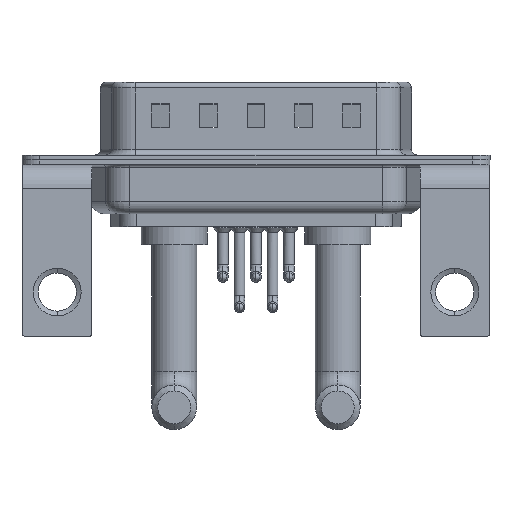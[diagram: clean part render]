
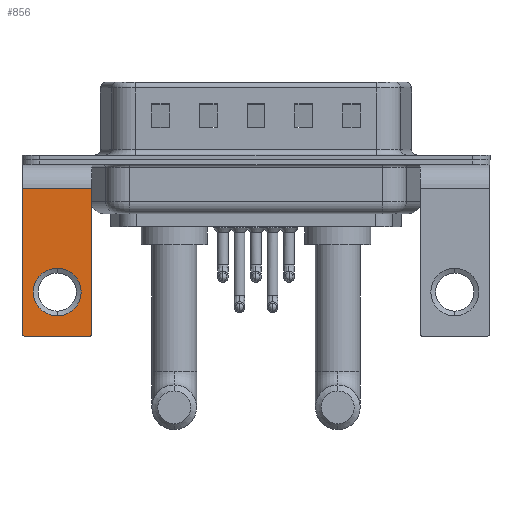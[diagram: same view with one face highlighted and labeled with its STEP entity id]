
A CAD part, front view. The second image highlights one B-rep face of the part: STEP entity #856.
In plain terms, the highlighted planar face has unit normal (0, -1, 0).
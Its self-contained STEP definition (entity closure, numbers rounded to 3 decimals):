
#97 = CARTESIAN_POINT ( 'NONE',  ( -2.65, -6.25, -14.55 ) ) ;
#414 = AXIS2_PLACEMENT_3D ( 'NONE', #17621, #9198, #20740 ) ;
#856 = ADVANCED_FACE ( 'NONE', ( #18692, #6859 ), #3530, .F. ) ;
#1128 = LINE ( 'NONE', #6307, #4351 ) ;
#1333 = EDGE_CURVE ( 'NONE', #2789, #5580, #4740, .T. ) ;
#2203 = DIRECTION ( 'NONE',  ( 0., 0., -1. ) ) ;
#2789 = VERTEX_POINT ( 'NONE', #12906 ) ;
#2883 = CARTESIAN_POINT ( 'NONE',  ( 2.65, -6.25, -14.55 ) ) ;
#3530 = PLANE ( 'NONE',  #4388 ) ;
#3622 = DIRECTION ( 'NONE',  ( 0., -1., 0. ) ) ;
#3652 = DIRECTION ( 'NONE',  ( 0., 0., 1. ) ) ;
#4194 = CARTESIAN_POINT ( 'NONE',  ( 0., -6.25, -11.07 ) ) ;
#4195 = CARTESIAN_POINT ( 'NONE',  ( 2.65, -6.25, -14.8 ) ) ;
#4351 = VECTOR ( 'NONE', #12850, 1000. ) ;
#4388 = AXIS2_PLACEMENT_3D ( 'NONE', #10601, #6972, #3652 ) ;
#4590 = CARTESIAN_POINT ( 'NONE',  ( 0., -6.25, -13.07 ) ) ;
#4740 = CIRCLE ( 'NONE', #16411, 0.25 ) ;
#4962 = EDGE_CURVE ( 'NONE', #6471, #11011, #20034, .T. ) ;
#5580 = VERTEX_POINT ( 'NONE', #7177 ) ;
#5656 = VECTOR ( 'NONE', #13497, 1000. ) ;
#5809 = VERTEX_POINT ( 'NONE', #4590 ) ;
#5896 = ORIENTED_EDGE ( 'NONE', *, *, #1333, .T. ) ;
#6063 = DIRECTION ( 'NONE',  ( 0., 1., 0. ) ) ;
#6274 = ORIENTED_EDGE ( 'NONE', *, *, #7810, .T. ) ;
#6307 = CARTESIAN_POINT ( 'NONE',  ( 2.9, -6.25, -14.8 ) ) ;
#6374 = CIRCLE ( 'NONE', #11019, 0.25 ) ;
#6471 = VERTEX_POINT ( 'NONE', #13721 ) ;
#6859 = FACE_OUTER_BOUND ( 'NONE', #13781, .T. ) ;
#6972 = DIRECTION ( 'NONE',  ( 0., 1., 0. ) ) ;
#7177 = CARTESIAN_POINT ( 'NONE',  ( -2.65, -6.25, -14.8 ) ) ;
#7543 = DIRECTION ( 'NONE',  ( 0., 0., 1. ) ) ;
#7599 = ORIENTED_EDGE ( 'NONE', *, *, #4962, .T. ) ;
#7730 = CARTESIAN_POINT ( 'NONE',  ( 2.9, -6.25, -14.55 ) ) ;
#7810 = EDGE_CURVE ( 'NONE', #20673, #5809, #17030, .T. ) ;
#8917 = DIRECTION ( 'NONE',  ( 0., 0., 1. ) ) ;
#9020 = EDGE_LOOP ( 'NONE', ( #14146, #6274 ) ) ;
#9198 = DIRECTION ( 'NONE',  ( 0., 1., 0. ) ) ;
#9271 = LINE ( 'NONE', #20586, #17512 ) ;
#9598 = DIRECTION ( 'NONE',  ( 0., 0., 1. ) ) ;
#10452 = AXIS2_PLACEMENT_3D ( 'NONE', #4194, #6063, #9598 ) ;
#10601 = CARTESIAN_POINT ( 'NONE',  ( 2.9, -6.25, -2.4 ) ) ;
#11011 = VERTEX_POINT ( 'NONE', #17751 ) ;
#11019 = AXIS2_PLACEMENT_3D ( 'NONE', #2883, #21381, #7543 ) ;
#11727 = CARTESIAN_POINT ( 'NONE',  ( 2.9, -6.25, -2.4 ) ) ;
#11760 = EDGE_CURVE ( 'NONE', #17559, #5580, #1128, .T. ) ;
#11994 = DIRECTION ( 'NONE',  ( 0., 0., -1. ) ) ;
#12850 = DIRECTION ( 'NONE',  ( -1., 0., 0. ) ) ;
#12906 = CARTESIAN_POINT ( 'NONE',  ( -2.9, -6.25, -14.55 ) ) ;
#13293 = EDGE_CURVE ( 'NONE', #11011, #2789, #13332, .T. ) ;
#13332 = LINE ( 'NONE', #15012, #15685 ) ;
#13497 = DIRECTION ( 'NONE',  ( -1., 0., 0. ) ) ;
#13721 = CARTESIAN_POINT ( 'NONE',  ( 2.9, -6.25, -2.4 ) ) ;
#13781 = EDGE_LOOP ( 'NONE', ( #20682, #5896, #15995, #17247, #15216, #7599 ) ) ;
#14146 = ORIENTED_EDGE ( 'NONE', *, *, #16301, .T. ) ;
#14345 = CARTESIAN_POINT ( 'NONE',  ( 0., -6.25, -9.07 ) ) ;
#15012 = CARTESIAN_POINT ( 'NONE',  ( -2.9, -6.25, -2.4 ) ) ;
#15216 = ORIENTED_EDGE ( 'NONE', *, *, #17601, .F. ) ;
#15685 = VECTOR ( 'NONE', #11994, 1000. ) ;
#15995 = ORIENTED_EDGE ( 'NONE', *, *, #11760, .F. ) ;
#16228 = VERTEX_POINT ( 'NONE', #7730 ) ;
#16301 = EDGE_CURVE ( 'NONE', #5809, #20673, #20352, .T. ) ;
#16411 = AXIS2_PLACEMENT_3D ( 'NONE', #97, #3622, #8917 ) ;
#17030 = CIRCLE ( 'NONE', #414, 2. ) ;
#17247 = ORIENTED_EDGE ( 'NONE', *, *, #21812, .T. ) ;
#17512 = VECTOR ( 'NONE', #2203, 1000. ) ;
#17559 = VERTEX_POINT ( 'NONE', #4195 ) ;
#17601 = EDGE_CURVE ( 'NONE', #6471, #16228, #9271, .T. ) ;
#17621 = CARTESIAN_POINT ( 'NONE',  ( 0., -6.25, -11.07 ) ) ;
#17751 = CARTESIAN_POINT ( 'NONE',  ( -2.9, -6.25, -2.4 ) ) ;
#18692 = FACE_BOUND ( 'NONE', #9020, .T. ) ;
#20034 = LINE ( 'NONE', #11727, #5656 ) ;
#20352 = CIRCLE ( 'NONE', #10452, 2. ) ;
#20586 = CARTESIAN_POINT ( 'NONE',  ( 2.9, -6.25, -2.4 ) ) ;
#20673 = VERTEX_POINT ( 'NONE', #14345 ) ;
#20682 = ORIENTED_EDGE ( 'NONE', *, *, #13293, .T. ) ;
#20740 = DIRECTION ( 'NONE',  ( 0., 0., 1. ) ) ;
#21381 = DIRECTION ( 'NONE',  ( 0., -1., 0. ) ) ;
#21812 = EDGE_CURVE ( 'NONE', #17559, #16228, #6374, .T. ) ;
